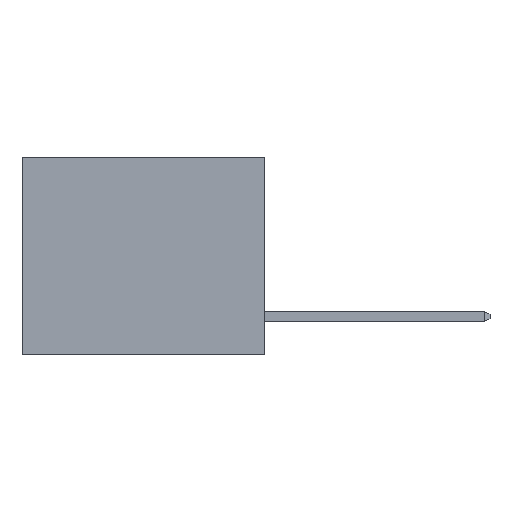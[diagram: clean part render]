
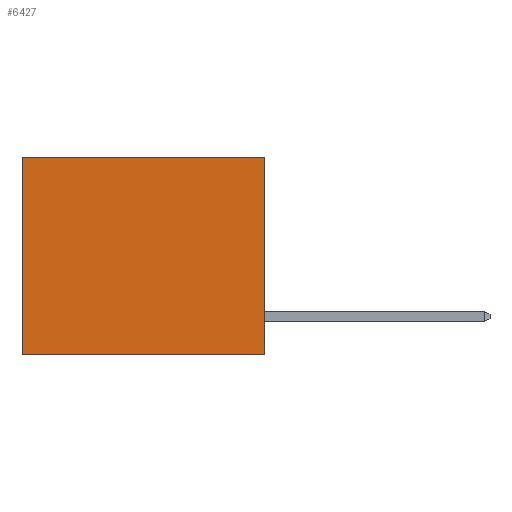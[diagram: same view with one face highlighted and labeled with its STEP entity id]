
A CAD part, left-side view. The second image highlights one B-rep face of the part: STEP entity #6427.
In plain terms, the highlighted planar face has unit normal (-1, 0, 0).
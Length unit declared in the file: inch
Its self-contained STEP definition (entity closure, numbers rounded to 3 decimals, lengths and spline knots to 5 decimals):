
#87 = FACE_OUTER_BOUND ( 'NONE', #7376, .T. ) ;
#384 = CARTESIAN_POINT ( 'NONE',  ( 0.3165, 0.6, -0.49 ) ) ;
#632 = ORIENTED_EDGE ( 'NONE', *, *, #6204, .F. ) ;
#641 = CARTESIAN_POINT ( 'NONE',  ( 0.3165, 0., -0.49 ) ) ;
#657 = DIRECTION ( 'NONE',  ( 0., 0., -1. ) ) ;
#1156 = LINE ( 'NONE', #641, #3820 ) ;
#1330 = CARTESIAN_POINT ( 'NONE',  ( 0.3165, 0.6, -0.49 ) ) ;
#1594 = LINE ( 'NONE', #1330, #5691 ) ;
#2179 = DIRECTION ( 'NONE',  ( 0., 0., -1. ) ) ;
#2689 = EDGE_CURVE ( 'NONE', #7615, #2794, #1156, .T. ) ;
#2794 = VERTEX_POINT ( 'NONE', #5306 ) ;
#2972 = DIRECTION ( 'NONE',  ( 0., 0., -1. ) ) ;
#3489 = VECTOR ( 'NONE', #5803, 39.37008 ) ;
#3820 = VECTOR ( 'NONE', #2972, 39.37008 ) ;
#3930 = AXIS2_PLACEMENT_3D ( 'NONE', #9987, #7662, #2179 ) ;
#4917 = CARTESIAN_POINT ( 'NONE',  ( 0.3165, 0.6, 0. ) ) ;
#5020 = CARTESIAN_POINT ( 'NONE',  ( 0.3165, 0., -0.49 ) ) ;
#5306 = CARTESIAN_POINT ( 'NONE',  ( 0.3165, 0., -0.49 ) ) ;
#5462 = ORIENTED_EDGE ( 'NONE', *, *, #8328, .T. ) ;
#5660 = ORIENTED_EDGE ( 'NONE', *, *, #2689, .F. ) ;
#5691 = VECTOR ( 'NONE', #657, 39.37008 ) ;
#5803 = DIRECTION ( 'NONE',  ( 0., 1., 0. ) ) ;
#6204 = EDGE_CURVE ( 'NONE', #2794, #7479, #9645, .T. ) ;
#6427 = ADVANCED_FACE ( 'NONE', ( #87 ), #8338, .F. ) ;
#6797 = CARTESIAN_POINT ( 'NONE',  ( 0.3165, 0., 0. ) ) ;
#7169 = DIRECTION ( 'NONE',  ( 0., 1., 0. ) ) ;
#7308 = EDGE_CURVE ( 'NONE', #7615, #7414, #7427, .T. ) ;
#7376 = EDGE_LOOP ( 'NONE', ( #5462, #632, #5660, #7433 ) ) ;
#7414 = VERTEX_POINT ( 'NONE', #4917 ) ;
#7427 = LINE ( 'NONE', #8658, #9724 ) ;
#7433 = ORIENTED_EDGE ( 'NONE', *, *, #7308, .T. ) ;
#7479 = VERTEX_POINT ( 'NONE', #384 ) ;
#7615 = VERTEX_POINT ( 'NONE', #6797 ) ;
#7662 = DIRECTION ( 'NONE',  ( 1., 0., 0. ) ) ;
#8328 = EDGE_CURVE ( 'NONE', #7414, #7479, #1594, .T. ) ;
#8338 = PLANE ( 'NONE',  #3930 ) ;
#8658 = CARTESIAN_POINT ( 'NONE',  ( 0.3165, 0., 0. ) ) ;
#9645 = LINE ( 'NONE', #5020, #3489 ) ;
#9724 = VECTOR ( 'NONE', #7169, 39.37008 ) ;
#9987 = CARTESIAN_POINT ( 'NONE',  ( 0.3165, 0., -0.49 ) ) ;
